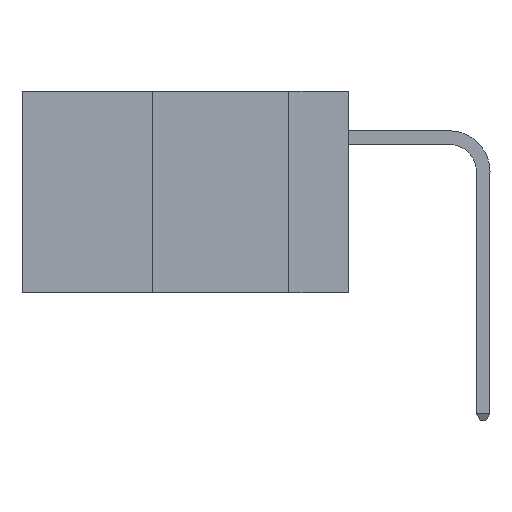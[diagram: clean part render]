
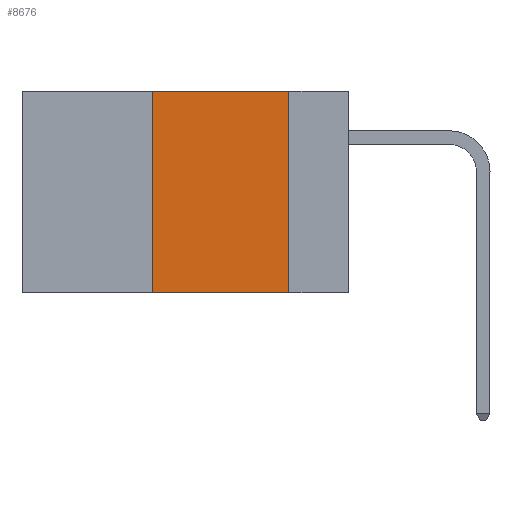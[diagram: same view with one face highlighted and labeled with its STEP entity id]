
A CAD part, left-side view. The second image highlights one B-rep face of the part: STEP entity #8676.
In plain terms, the highlighted planar face has unit normal (-1, 0, 0).
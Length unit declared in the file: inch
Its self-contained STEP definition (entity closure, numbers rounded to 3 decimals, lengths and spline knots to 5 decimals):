
#90 = VERTEX_POINT ( 'NONE', #5176 ) ;
#726 = VECTOR ( 'NONE', #10022, 39.37008 ) ;
#773 = CARTESIAN_POINT ( 'NONE',  ( 0., 0.6, 0. ) ) ;
#1581 = FACE_OUTER_BOUND ( 'NONE', #4072, .T. ) ;
#1654 = VECTOR ( 'NONE', #5535, 39.37008 ) ;
#1687 = DIRECTION ( 'NONE',  ( 0., 0., -1. ) ) ;
#3030 = DIRECTION ( 'NONE',  ( 0., 0., 1. ) ) ;
#3276 = ORIENTED_EDGE ( 'NONE', *, *, #7088, .F. ) ;
#3850 = LINE ( 'NONE', #11100, #726 ) ;
#3993 = DIRECTION ( 'NONE',  ( 1., 0., 0. ) ) ;
#4072 = EDGE_LOOP ( 'NONE', ( #12047, #3276, #7988, #17339 ) ) ;
#5134 = CARTESIAN_POINT ( 'NONE',  ( 0., 0.36, 0. ) ) ;
#5176 = CARTESIAN_POINT ( 'NONE',  ( 0., 0.11, -0.37 ) ) ;
#5431 = DIRECTION ( 'NONE',  ( 0., 0., -1. ) ) ;
#5535 = DIRECTION ( 'NONE',  ( 0., -1., 0. ) ) ;
#7088 = EDGE_CURVE ( 'NONE', #18249, #19369, #18405, .T. ) ;
#7497 = VERTEX_POINT ( 'NONE', #18064 ) ;
#7988 = ORIENTED_EDGE ( 'NONE', *, *, #8898, .F. ) ;
#8505 = AXIS2_PLACEMENT_3D ( 'NONE', #773, #3993, #5431 ) ;
#8676 = ADVANCED_FACE ( 'NONE', ( #1581 ), #10109, .F. ) ;
#8871 = VECTOR ( 'NONE', #3030, 39.37008 ) ;
#8898 = EDGE_CURVE ( 'NONE', #7497, #18249, #12783, .T. ) ;
#10022 = DIRECTION ( 'NONE',  ( 0., -1., 0. ) ) ;
#10109 = PLANE ( 'NONE',  #8505 ) ;
#11100 = CARTESIAN_POINT ( 'NONE',  ( 0., 0.6, -0.37 ) ) ;
#12047 = ORIENTED_EDGE ( 'NONE', *, *, #14970, .F. ) ;
#12632 = VECTOR ( 'NONE', #1687, 39.37008 ) ;
#12783 = LINE ( 'NONE', #15583, #8871 ) ;
#13776 = EDGE_CURVE ( 'NONE', #7497, #90, #3850, .T. ) ;
#14341 = LINE ( 'NONE', #17165, #12632 ) ;
#14970 = EDGE_CURVE ( 'NONE', #19369, #90, #14341, .T. ) ;
#15489 = CARTESIAN_POINT ( 'NONE',  ( 0., 0.6, 0. ) ) ;
#15583 = CARTESIAN_POINT ( 'NONE',  ( 0., 0.36, 0. ) ) ;
#16000 = CARTESIAN_POINT ( 'NONE',  ( 0., 0.11, 0. ) ) ;
#17165 = CARTESIAN_POINT ( 'NONE',  ( 0., 0.11, 0. ) ) ;
#17339 = ORIENTED_EDGE ( 'NONE', *, *, #13776, .T. ) ;
#18064 = CARTESIAN_POINT ( 'NONE',  ( 0., 0.36, -0.37 ) ) ;
#18249 = VERTEX_POINT ( 'NONE', #5134 ) ;
#18405 = LINE ( 'NONE', #15489, #1654 ) ;
#19369 = VERTEX_POINT ( 'NONE', #16000 ) ;
